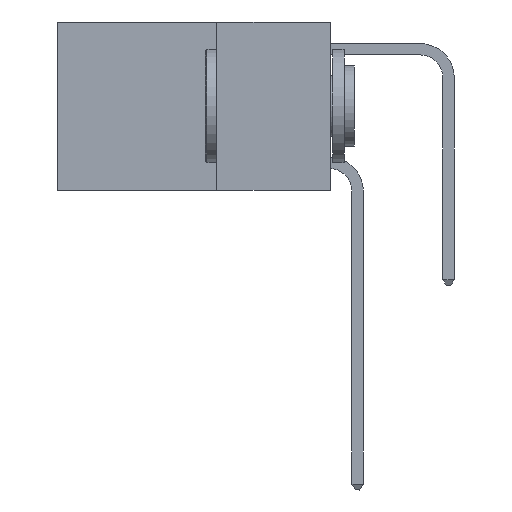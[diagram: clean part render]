
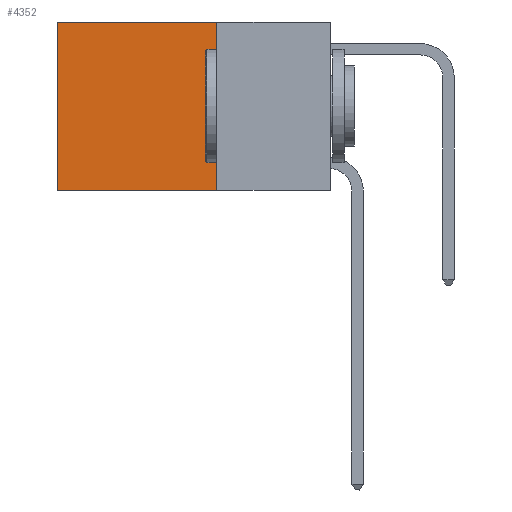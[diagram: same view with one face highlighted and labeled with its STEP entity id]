
A CAD part, left-side view. The second image highlights one B-rep face of the part: STEP entity #4352.
In plain terms, the highlighted planar face has unit normal (-1, 0, 0).
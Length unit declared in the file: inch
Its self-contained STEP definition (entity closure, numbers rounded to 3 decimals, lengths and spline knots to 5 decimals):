
#929 = LINE ( 'NONE', #11326, #15586 ) ;
#1456 = LINE ( 'NONE', #5255, #7797 ) ;
#1588 = DIRECTION ( 'NONE',  ( 0., 1., 0. ) ) ;
#3599 = CARTESIAN_POINT ( 'NONE',  ( 0.2625, 0.6, -0.37 ) ) ;
#4352 = ADVANCED_FACE ( 'NONE', ( #23423 ), #7483, .F. ) ;
#5255 = CARTESIAN_POINT ( 'NONE',  ( 0.2625, 0.25, 0. ) ) ;
#7193 = VERTEX_POINT ( 'NONE', #8509 ) ;
#7281 = EDGE_CURVE ( 'NONE', #23338, #24158, #1456, .T. ) ;
#7483 = PLANE ( 'NONE',  #17113 ) ;
#7797 = VECTOR ( 'NONE', #1588, 39.37008 ) ;
#7879 = DIRECTION ( 'NONE',  ( 0., 0., -1. ) ) ;
#8509 = CARTESIAN_POINT ( 'NONE',  ( 0.2625, 0.25, -0.37 ) ) ;
#8576 = ORIENTED_EDGE ( 'NONE', *, *, #7281, .T. ) ;
#8738 = DIRECTION ( 'NONE',  ( 0., 0., -1. ) ) ;
#10092 = EDGE_CURVE ( 'NONE', #24158, #14189, #13688, .T. ) ;
#10390 = EDGE_CURVE ( 'NONE', #7193, #14189, #929, .T. ) ;
#10791 = ORIENTED_EDGE ( 'NONE', *, *, #23113, .F. ) ;
#11157 = ORIENTED_EDGE ( 'NONE', *, *, #10390, .F. ) ;
#11326 = CARTESIAN_POINT ( 'NONE',  ( 0.2625, 0.25, -0.37 ) ) ;
#11936 = CARTESIAN_POINT ( 'NONE',  ( 0.2625, 0.25, 0. ) ) ;
#13443 = CARTESIAN_POINT ( 'NONE',  ( 0.2625, 0.25, 0. ) ) ;
#13555 = CARTESIAN_POINT ( 'NONE',  ( 0.2625, 0.6, 0. ) ) ;
#13688 = LINE ( 'NONE', #15639, #17502 ) ;
#14189 = VERTEX_POINT ( 'NONE', #3599 ) ;
#15089 = VECTOR ( 'NONE', #8738, 39.37008 ) ;
#15586 = VECTOR ( 'NONE', #22752, 39.37008 ) ;
#15639 = CARTESIAN_POINT ( 'NONE',  ( 0.2625, 0.6, 0. ) ) ;
#15859 = EDGE_LOOP ( 'NONE', ( #19853, #11157, #10791, #8576 ) ) ;
#17113 = AXIS2_PLACEMENT_3D ( 'NONE', #13443, #23173, #7879 ) ;
#17502 = VECTOR ( 'NONE', #21469, 39.37008 ) ;
#19108 = CARTESIAN_POINT ( 'NONE',  ( 0.2625, 0.25, 0. ) ) ;
#19853 = ORIENTED_EDGE ( 'NONE', *, *, #10092, .T. ) ;
#21469 = DIRECTION ( 'NONE',  ( 0., 0., -1. ) ) ;
#22752 = DIRECTION ( 'NONE',  ( 0., 1., 0. ) ) ;
#23113 = EDGE_CURVE ( 'NONE', #23338, #7193, #24442, .T. ) ;
#23173 = DIRECTION ( 'NONE',  ( 1., 0., 0. ) ) ;
#23338 = VERTEX_POINT ( 'NONE', #11936 ) ;
#23423 = FACE_OUTER_BOUND ( 'NONE', #15859, .T. ) ;
#24158 = VERTEX_POINT ( 'NONE', #13555 ) ;
#24442 = LINE ( 'NONE', #19108, #15089 ) ;
